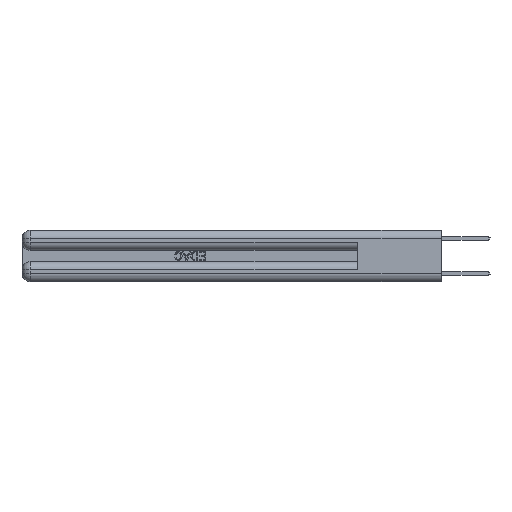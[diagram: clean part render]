
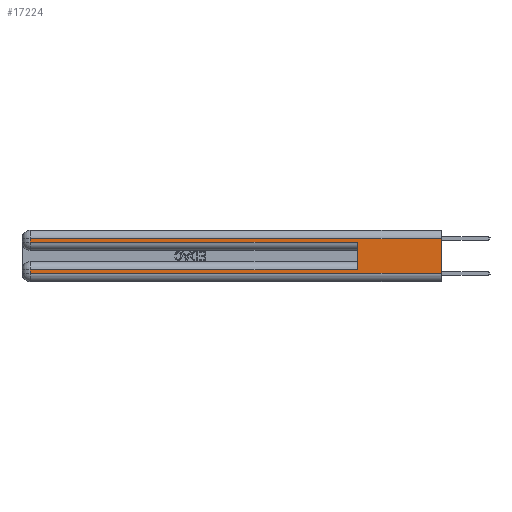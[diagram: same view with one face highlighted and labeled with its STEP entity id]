
A CAD part, left-side view. The second image highlights one B-rep face of the part: STEP entity #17224.
In plain terms, the highlighted planar face has unit normal (-1, 0, 0).
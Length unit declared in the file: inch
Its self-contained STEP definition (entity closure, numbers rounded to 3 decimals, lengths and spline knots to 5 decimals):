
#214 = CARTESIAN_POINT ( 'NONE',  ( 0., 2.94, 0.285 ) ) ;
#529 = EDGE_CURVE ( 'NONE', #28940, #27319, #10827, .T. ) ;
#623 = AXIS2_PLACEMENT_3D ( 'NONE', #2047, #11110, #20205 ) ;
#697 = LINE ( 'NONE', #15886, #24776 ) ;
#1310 = VECTOR ( 'NONE', #17411, 39.37008 ) ;
#1610 = CARTESIAN_POINT ( 'NONE',  ( 0., 2.94, 0.37 ) ) ;
#2047 = CARTESIAN_POINT ( 'NONE',  ( 0., 0., 0.37 ) ) ;
#2054 = ORIENTED_EDGE ( 'NONE', *, *, #3369, .F. ) ;
#2648 = VECTOR ( 'NONE', #25326, 39.37008 ) ;
#2800 = CARTESIAN_POINT ( 'NONE',  ( 0., 0., 0.285 ) ) ;
#3017 = LINE ( 'NONE', #28050, #27250 ) ;
#3369 = EDGE_CURVE ( 'NONE', #21903, #8699, #8753, .T. ) ;
#3633 = EDGE_CURVE ( 'NONE', #5092, #17787, #10219, .T. ) ;
#3912 = LINE ( 'NONE', #10479, #16578 ) ;
#4994 = CARTESIAN_POINT ( 'NONE',  ( 0., 0., 0.31 ) ) ;
#5092 = VERTEX_POINT ( 'NONE', #4994 ) ;
#6052 = EDGE_LOOP ( 'NONE', ( #27394, #21833, #25794, #29254, #2054, #26115, #14487, #18413 ) ) ;
#7761 = EDGE_CURVE ( 'NONE', #11173, #19852, #7875, .T. ) ;
#7875 = LINE ( 'NONE', #16378, #2648 ) ;
#8298 = VECTOR ( 'NONE', #11417, 39.37008 ) ;
#8394 = CARTESIAN_POINT ( 'NONE',  ( 0., 0.6, 0.285 ) ) ;
#8699 = VERTEX_POINT ( 'NONE', #8394 ) ;
#8753 = LINE ( 'NONE', #17844, #1310 ) ;
#9781 = DIRECTION ( 'NONE',  ( 0., 1., 0. ) ) ;
#10219 = LINE ( 'NONE', #28424, #11778 ) ;
#10479 = CARTESIAN_POINT ( 'NONE',  ( 0., 0., 0.06 ) ) ;
#10706 = EDGE_CURVE ( 'NONE', #21903, #11173, #3017, .T. ) ;
#10827 = LINE ( 'NONE', #1610, #12345 ) ;
#11110 = DIRECTION ( 'NONE',  ( 1., 0., 0. ) ) ;
#11173 = VERTEX_POINT ( 'NONE', #16537 ) ;
#11417 = DIRECTION ( 'NONE',  ( 0., -1., 0. ) ) ;
#11564 = EDGE_CURVE ( 'NONE', #27319, #8699, #11886, .T. ) ;
#11778 = VECTOR ( 'NONE', #25593, 39.37008 ) ;
#11788 = CARTESIAN_POINT ( 'NONE',  ( 0., 2.94, 0.31 ) ) ;
#11886 = LINE ( 'NONE', #2800, #8298 ) ;
#12345 = VECTOR ( 'NONE', #12760, 39.37008 ) ;
#12648 = EDGE_CURVE ( 'NONE', #5092, #28940, #697, .T. ) ;
#12760 = DIRECTION ( 'NONE',  ( 0., 0., -1. ) ) ;
#14487 = ORIENTED_EDGE ( 'NONE', *, *, #7761, .T. ) ;
#15091 = DIRECTION ( 'NONE',  ( 0., -1., 0. ) ) ;
#15143 = CARTESIAN_POINT ( 'NONE',  ( 0., 0.6, 0.085 ) ) ;
#15886 = CARTESIAN_POINT ( 'NONE',  ( 0., 0., 0.31 ) ) ;
#16378 = CARTESIAN_POINT ( 'NONE',  ( 0., 2.94, 0.37 ) ) ;
#16537 = CARTESIAN_POINT ( 'NONE',  ( 0., 2.94, 0.085 ) ) ;
#16578 = VECTOR ( 'NONE', #15091, 39.37008 ) ;
#17224 = ADVANCED_FACE ( 'NONE', ( #26778 ), #19921, .F. ) ;
#17411 = DIRECTION ( 'NONE',  ( 0., 0., 1. ) ) ;
#17736 = CARTESIAN_POINT ( 'NONE',  ( 0., 2.94, 0.06 ) ) ;
#17787 = VERTEX_POINT ( 'NONE', #18799 ) ;
#17844 = CARTESIAN_POINT ( 'NONE',  ( 0., 0.6, 0.145 ) ) ;
#18413 = ORIENTED_EDGE ( 'NONE', *, *, #24399, .T. ) ;
#18799 = CARTESIAN_POINT ( 'NONE',  ( 0., 0., 0.06 ) ) ;
#19852 = VERTEX_POINT ( 'NONE', #17736 ) ;
#19921 = PLANE ( 'NONE',  #623 ) ;
#20205 = DIRECTION ( 'NONE',  ( 0., 0., -1. ) ) ;
#21833 = ORIENTED_EDGE ( 'NONE', *, *, #12648, .T. ) ;
#21903 = VERTEX_POINT ( 'NONE', #15143 ) ;
#24399 = EDGE_CURVE ( 'NONE', #19852, #17787, #3912, .T. ) ;
#24776 = VECTOR ( 'NONE', #9781, 39.37008 ) ;
#25326 = DIRECTION ( 'NONE',  ( 0., 0., -1. ) ) ;
#25593 = DIRECTION ( 'NONE',  ( 0., 0., -1. ) ) ;
#25794 = ORIENTED_EDGE ( 'NONE', *, *, #529, .T. ) ;
#26115 = ORIENTED_EDGE ( 'NONE', *, *, #10706, .T. ) ;
#26778 = FACE_OUTER_BOUND ( 'NONE', #6052, .T. ) ;
#27250 = VECTOR ( 'NONE', #27450, 39.37008 ) ;
#27319 = VERTEX_POINT ( 'NONE', #214 ) ;
#27394 = ORIENTED_EDGE ( 'NONE', *, *, #3633, .F. ) ;
#27450 = DIRECTION ( 'NONE',  ( 0., 1., 0. ) ) ;
#28050 = CARTESIAN_POINT ( 'NONE',  ( 0., 0., 0.085 ) ) ;
#28424 = CARTESIAN_POINT ( 'NONE',  ( 0., 0., 0.37 ) ) ;
#28940 = VERTEX_POINT ( 'NONE', #11788 ) ;
#29254 = ORIENTED_EDGE ( 'NONE', *, *, #11564, .T. ) ;
